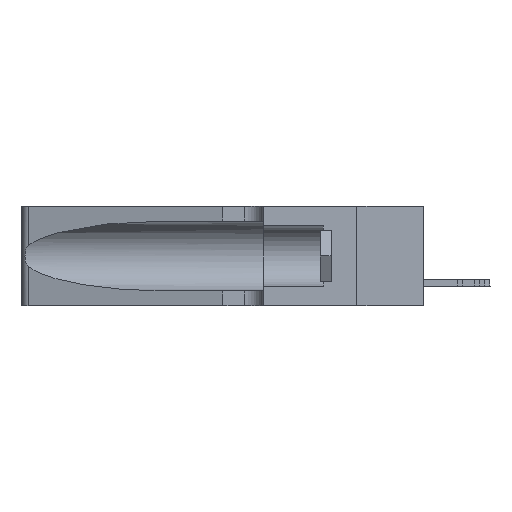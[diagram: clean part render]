
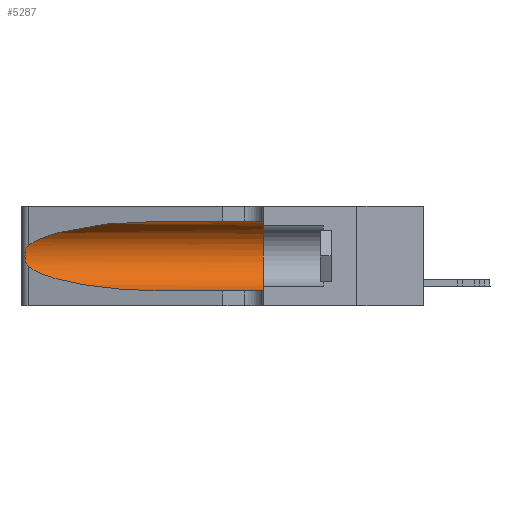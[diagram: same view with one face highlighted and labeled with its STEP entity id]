
A CAD part, left-side view. The second image highlights one B-rep face of the part: STEP entity #5287.
In plain terms, the highlighted cylindrical face has radius 3.308 mm (diameter 6.617 mm), a partial arc.
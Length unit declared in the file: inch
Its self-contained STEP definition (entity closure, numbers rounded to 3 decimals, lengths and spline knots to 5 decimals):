
#860 = EDGE_CURVE ( 'NONE', #51132, #42292, #32822, .T. ) ;
#1150 = CARTESIAN_POINT ( 'NONE',  ( 0.25555, 1.22994, 0.2215 ) ) ;
#2221 = CARTESIAN_POINT ( 'NONE',  ( 0.18966, 0.96281, 0.31525 ) ) ;
#2537 = CYLINDRICAL_SURFACE ( 'NONE', #47922, 0.13025 ) ;
#5206 = EDGE_CURVE ( 'NONE', #50433, #20328, #15003, .T. ) ;
#5287 = ADVANCED_FACE ( 'NONE', ( #23757 ), #2537, .F. ) ;
#6541 = CARTESIAN_POINT ( 'NONE',  ( 0.26075, 1.23896, 0.19203 ) ) ;
#6915 = CARTESIAN_POINT ( 'NONE',  ( 0.25555, 1.22993, 0.14849 ) ) ;
#7559 = CARTESIAN_POINT ( 'NONE',  ( 0.25487, 1.22718, 0.22369 ) ) ;
#9197 = CARTESIAN_POINT ( 'NONE',  ( 0.1305, 0.72297, 0.05475 ) ) ;
#9841 = CARTESIAN_POINT ( 'NONE',  ( 0.1305, 0.72297, 0.31525 ) ) ;
#10233 = CARTESIAN_POINT ( 'NONE',  ( 0.25487, 1.22718, 0.22369 ) ) ;
#10846 = CARTESIAN_POINT ( 'NONE',  ( 0.1305, 0.35, 0.185 ) ) ;
#10883 =( BOUNDED_CURVE ( )  B_SPLINE_CURVE ( 3, ( #9841, #2221, #17830, #10233 ),
 .UNSPECIFIED., .F., .F. ) 
 B_SPLINE_CURVE_WITH_KNOTS ( ( 4, 4 ),
 ( 1.5708, 2.84003 ),
 .UNSPECIFIED. ) 
 CURVE ( )  GEOMETRIC_REPRESENTATION_ITEM ( )  RATIONAL_B_SPLINE_CURVE ( ( 1., 0.87, 0.87, 1. ) ) 
 REPRESENTATION_ITEM ( '' )  );
#11715 = VECTOR ( 'NONE', #50756, 39.37008 ) ;
#15003 = LINE ( 'NONE', #50720, #47519 ) ;
#15469 = ORIENTED_EDGE ( 'NONE', *, *, #35375, .T. ) ;
#17830 = CARTESIAN_POINT ( 'NONE',  ( 0.2373, 1.15595, 0.28018 ) ) ;
#18051 = DIRECTION ( 'NONE',  ( 0., 1., 0. ) ) ;
#18621 = CARTESIAN_POINT ( 'NONE',  ( 0.18966, 0.96281, 0.05475 ) ) ;
#19015 = EDGE_CURVE ( 'NONE', #42292, #31802, #22226, .T. ) ;
#19176 = B_SPLINE_CURVE_WITH_KNOTS ( 'NONE', 3,
 ( #33470, #1150, #34241, #42275, #26375, #26553, #6541, #40170, #43870, #35996, #46658, #26745, #6915, #24701 ),
 .UNSPECIFIED., .F., .F.,
 ( 4, 2, 2, 2, 2, 2, 4 ),
 ( 0., 0.00027, 0.00053, 0.00107, 0.0016, 0.00187, 0.00214 ),
 .UNSPECIFIED. ) ;
#19246 = AXIS2_PLACEMENT_3D ( 'NONE', #10846, #18051, #38782 ) ;
#19835 = CARTESIAN_POINT ( 'NONE',  ( 0.1305, 0.35, 0.31525 ) ) ;
#20328 = VERTEX_POINT ( 'NONE', #19835 ) ;
#22226 = LINE ( 'NONE', #22788, #11715 ) ;
#22636 = CARTESIAN_POINT ( 'NONE',  ( 0.1305, 0.72297, 0.05475 ) ) ;
#22788 = CARTESIAN_POINT ( 'NONE',  ( 0.1305, 1.61858, 0.05475 ) ) ;
#23757 = FACE_OUTER_BOUND ( 'NONE', #51575, .T. ) ;
#24701 = CARTESIAN_POINT ( 'NONE',  ( 0.25487, 1.22718, 0.14631 ) ) ;
#25609 = ORIENTED_EDGE ( 'NONE', *, *, #5206, .F. ) ;
#26375 = CARTESIAN_POINT ( 'NONE',  ( 0.25854, 1.2359, 0.20912 ) ) ;
#26393 = ORIENTED_EDGE ( 'NONE', *, *, #19015, .T. ) ;
#26553 = CARTESIAN_POINT ( 'NONE',  ( 0.26018, 1.23835, 0.19895 ) ) ;
#26745 = CARTESIAN_POINT ( 'NONE',  ( 0.25639, 1.23186, 0.15144 ) ) ;
#26808 = DIRECTION ( 'NONE',  ( 0., -1., 0. ) ) ;
#31080 = CARTESIAN_POINT ( 'NONE',  ( 0.1305, 0.35, 0.05475 ) ) ;
#31802 = VERTEX_POINT ( 'NONE', #31080 ) ;
#32344 = DIRECTION ( 'NONE',  ( 0., -1., 0. ) ) ;
#32497 = CARTESIAN_POINT ( 'NONE',  ( 0.1305, 1.61858, 0.185 ) ) ;
#32822 =( BOUNDED_CURVE ( )  B_SPLINE_CURVE ( 3, ( #39133, #38579, #18621, #22636 ),
 .UNSPECIFIED., .F., .T. ) 
 B_SPLINE_CURVE_WITH_KNOTS ( ( 4, 4 ),
 ( 3.44316, 4.71239 ),
 .UNSPECIFIED. ) 
 CURVE ( )  GEOMETRIC_REPRESENTATION_ITEM ( )  RATIONAL_B_SPLINE_CURVE ( ( 1., 0.87, 0.87, 1. ) ) 
 REPRESENTATION_ITEM ( '' )  );
#33470 = CARTESIAN_POINT ( 'NONE',  ( 0.25487, 1.22718, 0.22369 ) ) ;
#34241 = CARTESIAN_POINT ( 'NONE',  ( 0.25639, 1.23184, 0.21858 ) ) ;
#35375 = EDGE_CURVE ( 'NONE', #50433, #41435, #10883, .T. ) ;
#35996 = CARTESIAN_POINT ( 'NONE',  ( 0.25856, 1.23593, 0.16098 ) ) ;
#37438 = EDGE_CURVE ( 'NONE', #20328, #31802, #42064, .T. ) ;
#38370 = EDGE_CURVE ( 'NONE', #41435, #51132, #19176, .T. ) ;
#38402 = CARTESIAN_POINT ( 'NONE',  ( 0.1305, 0.72297, 0.31525 ) ) ;
#38579 = CARTESIAN_POINT ( 'NONE',  ( 0.2373, 1.15595, 0.08982 ) ) ;
#38782 = DIRECTION ( 'NONE',  ( 0., 0., 1. ) ) ;
#39133 = CARTESIAN_POINT ( 'NONE',  ( 0.25487, 1.22718, 0.14631 ) ) ;
#40170 = CARTESIAN_POINT ( 'NONE',  ( 0.26075, 1.23896, 0.178 ) ) ;
#41161 = CARTESIAN_POINT ( 'NONE',  ( 0.25487, 1.22718, 0.14631 ) ) ;
#41435 = VERTEX_POINT ( 'NONE', #7559 ) ;
#42064 = CIRCLE ( 'NONE', #19246, 0.13025 ) ;
#42275 = CARTESIAN_POINT ( 'NONE',  ( 0.25787, 1.23484, 0.2124 ) ) ;
#42292 = VERTEX_POINT ( 'NONE', #9197 ) ;
#43870 = CARTESIAN_POINT ( 'NONE',  ( 0.26017, 1.23833, 0.17102 ) ) ;
#43929 = ORIENTED_EDGE ( 'NONE', *, *, #37438, .F. ) ;
#46658 = CARTESIAN_POINT ( 'NONE',  ( 0.25789, 1.23486, 0.15765 ) ) ;
#47519 = VECTOR ( 'NONE', #26808, 39.37008 ) ;
#47922 = AXIS2_PLACEMENT_3D ( 'NONE', #32497, #32344, #49503 ) ;
#48336 = ORIENTED_EDGE ( 'NONE', *, *, #860, .T. ) ;
#49503 = DIRECTION ( 'NONE',  ( 0., 0., -1. ) ) ;
#50433 = VERTEX_POINT ( 'NONE', #38402 ) ;
#50720 = CARTESIAN_POINT ( 'NONE',  ( 0.1305, 1.61858, 0.31525 ) ) ;
#50756 = DIRECTION ( 'NONE',  ( 0., -1., 0. ) ) ;
#51132 = VERTEX_POINT ( 'NONE', #41161 ) ;
#51390 = ORIENTED_EDGE ( 'NONE', *, *, #38370, .T. ) ;
#51575 = EDGE_LOOP ( 'NONE', ( #15469, #51390, #48336, #26393, #43929, #25609 ) ) ;
